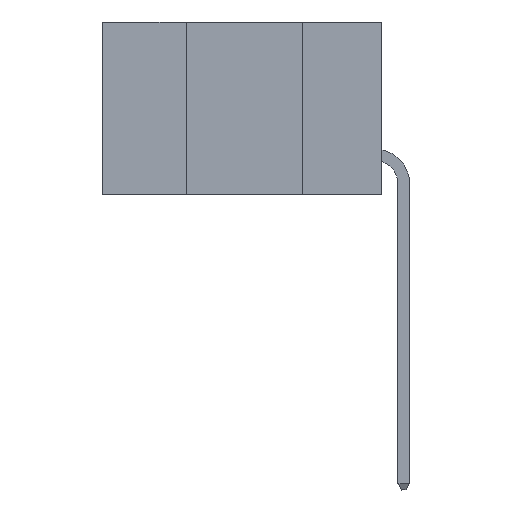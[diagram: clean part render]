
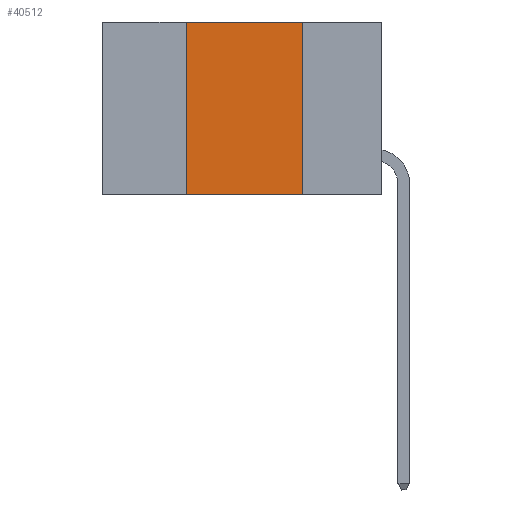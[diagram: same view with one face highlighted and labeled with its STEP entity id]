
A CAD part, left-side view. The second image highlights one B-rep face of the part: STEP entity #40512.
In plain terms, the highlighted planar face has unit normal (-1, 0, 0).
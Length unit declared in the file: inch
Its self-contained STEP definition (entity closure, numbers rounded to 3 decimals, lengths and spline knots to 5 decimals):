
#4384 = CARTESIAN_POINT ( 'NONE',  ( 0., 0.17, -0.37 ) ) ;
#4705 = LINE ( 'NONE', #21077, #28808 ) ;
#4719 = VERTEX_POINT ( 'NONE', #30123 ) ;
#8121 = LINE ( 'NONE', #14477, #44123 ) ;
#8805 = EDGE_CURVE ( 'NONE', #4719, #11836, #43434, .T. ) ;
#8993 = EDGE_LOOP ( 'NONE', ( #18304, #40233, #45090, #23430 ) ) ;
#10315 = VERTEX_POINT ( 'NONE', #10478 ) ;
#10478 = CARTESIAN_POINT ( 'NONE',  ( 0., 0.42, -0.37 ) ) ;
#10699 = AXIS2_PLACEMENT_3D ( 'NONE', #13267, #23791, #27358 ) ;
#11836 = VERTEX_POINT ( 'NONE', #4384 ) ;
#13267 = CARTESIAN_POINT ( 'NONE',  ( 0., 0.6, 0. ) ) ;
#14477 = CARTESIAN_POINT ( 'NONE',  ( 0., 0.6, -0.37 ) ) ;
#17854 = EDGE_CURVE ( 'NONE', #10315, #30697, #22123, .T. ) ;
#17938 = DIRECTION ( 'NONE',  ( 0., -1., 0. ) ) ;
#18304 = ORIENTED_EDGE ( 'NONE', *, *, #8805, .F. ) ;
#21077 = CARTESIAN_POINT ( 'NONE',  ( 0., 0.6, 0. ) ) ;
#22123 = LINE ( 'NONE', #22871, #33857 ) ;
#22871 = CARTESIAN_POINT ( 'NONE',  ( 0., 0.42, 0. ) ) ;
#23430 = ORIENTED_EDGE ( 'NONE', *, *, #46207, .T. ) ;
#23539 = DIRECTION ( 'NONE',  ( 0., 0., -1. ) ) ;
#23791 = DIRECTION ( 'NONE',  ( 1., 0., 0. ) ) ;
#25147 = VECTOR ( 'NONE', #23539, 39.37008 ) ;
#27358 = DIRECTION ( 'NONE',  ( 0., 0., -1. ) ) ;
#28808 = VECTOR ( 'NONE', #42404, 39.37008 ) ;
#30123 = CARTESIAN_POINT ( 'NONE',  ( 0., 0.17, 0. ) ) ;
#30697 = VERTEX_POINT ( 'NONE', #37046 ) ;
#33857 = VECTOR ( 'NONE', #40571, 39.37008 ) ;
#37046 = CARTESIAN_POINT ( 'NONE',  ( 0., 0.42, 0. ) ) ;
#40233 = ORIENTED_EDGE ( 'NONE', *, *, #46589, .F. ) ;
#40512 = ADVANCED_FACE ( 'NONE', ( #40790 ), #45941, .F. ) ;
#40571 = DIRECTION ( 'NONE',  ( 0., 0., 1. ) ) ;
#40790 = FACE_OUTER_BOUND ( 'NONE', #8993, .T. ) ;
#42404 = DIRECTION ( 'NONE',  ( 0., -1., 0. ) ) ;
#43434 = LINE ( 'NONE', #45053, #25147 ) ;
#44123 = VECTOR ( 'NONE', #17938, 39.37008 ) ;
#45053 = CARTESIAN_POINT ( 'NONE',  ( 0., 0.17, 0. ) ) ;
#45090 = ORIENTED_EDGE ( 'NONE', *, *, #17854, .F. ) ;
#45941 = PLANE ( 'NONE',  #10699 ) ;
#46207 = EDGE_CURVE ( 'NONE', #10315, #11836, #8121, .T. ) ;
#46589 = EDGE_CURVE ( 'NONE', #30697, #4719, #4705, .T. ) ;
